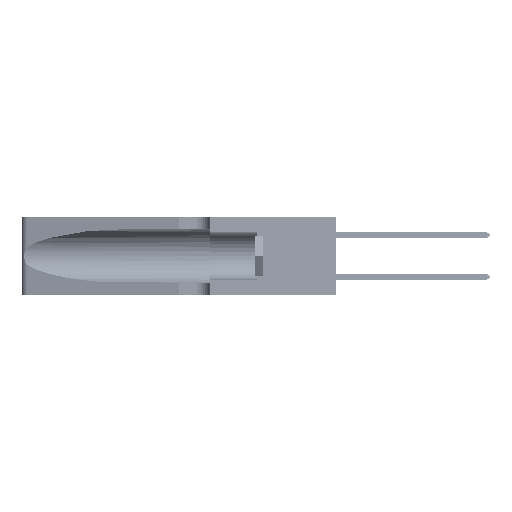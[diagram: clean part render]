
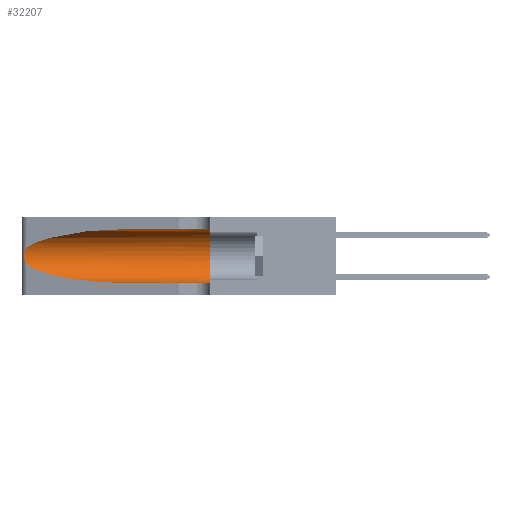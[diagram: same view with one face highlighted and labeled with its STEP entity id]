
A CAD part, left-side view. The second image highlights one B-rep face of the part: STEP entity #32207.
In plain terms, the highlighted cylindrical face has radius 3.308 mm (diameter 6.617 mm), a partial arc.
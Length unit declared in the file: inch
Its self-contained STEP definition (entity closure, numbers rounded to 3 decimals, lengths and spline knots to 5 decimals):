
#1120 = CARTESIAN_POINT ( 'NONE',  ( 0.2373, 1.15595, 0.28018 ) ) ;
#2600 = VERTEX_POINT ( 'NONE', #28276 ) ;
#2795 = EDGE_CURVE ( 'NONE', #25379, #2600, #51472, .T. ) ;
#2971 = ORIENTED_EDGE ( 'NONE', *, *, #19829, .F. ) ;
#3162 = CARTESIAN_POINT ( 'NONE',  ( 0.1305, 0.72297, 0.31525 ) ) ;
#4078 = ORIENTED_EDGE ( 'NONE', *, *, #41213, .T. ) ;
#4737 = DIRECTION ( 'NONE',  ( 0., 0., -1. ) ) ;
#5850 = CARTESIAN_POINT ( 'NONE',  ( 0.1305, 1.61858, 0.05475 ) ) ;
#6497 = CARTESIAN_POINT ( 'NONE',  ( 0.25639, 1.23184, 0.21858 ) ) ;
#6669 = CARTESIAN_POINT ( 'NONE',  ( 0.26075, 1.23896, 0.19203 ) ) ;
#8155 = CARTESIAN_POINT ( 'NONE',  ( 0.25487, 1.22718, 0.22369 ) ) ;
#8171 = CARTESIAN_POINT ( 'NONE',  ( 0.25487, 1.22718, 0.14631 ) ) ;
#10570 = CARTESIAN_POINT ( 'NONE',  ( 0.26018, 1.23835, 0.19895 ) ) ;
#12343 =( BOUNDED_CURVE ( )  B_SPLINE_CURVE ( 3, ( #16083, #21004, #1120, #45771 ),
 .UNSPECIFIED., .F., .T. ) 
 B_SPLINE_CURVE_WITH_KNOTS ( ( 4, 4 ),
 ( 1.5708, 2.84003 ),
 .UNSPECIFIED. ) 
 CURVE ( )  GEOMETRIC_REPRESENTATION_ITEM ( )  RATIONAL_B_SPLINE_CURVE ( ( 1., 0.87, 0.87, 1. ) ) 
 REPRESENTATION_ITEM ( '' )  );
#13330 = EDGE_LOOP ( 'NONE', ( #48797, #4078, #43429, #39478, #13455, #2971 ) ) ;
#13455 = ORIENTED_EDGE ( 'NONE', *, *, #2795, .F. ) ;
#14400 = CARTESIAN_POINT ( 'NONE',  ( 0.25487, 1.22718, 0.14631 ) ) ;
#14750 = CARTESIAN_POINT ( 'NONE',  ( 0.25555, 1.22994, 0.2215 ) ) ;
#14924 = CARTESIAN_POINT ( 'NONE',  ( 0.25487, 1.22718, 0.22369 ) ) ;
#16083 = CARTESIAN_POINT ( 'NONE',  ( 0.1305, 0.72297, 0.31525 ) ) ;
#17187 = VERTEX_POINT ( 'NONE', #3162 ) ;
#18982 = EDGE_CURVE ( 'NONE', #36548, #25638, #21703, .T. ) ;
#19829 = EDGE_CURVE ( 'NONE', #17187, #25379, #41629, .T. ) ;
#20240 = VECTOR ( 'NONE', #37278, 39.37008 ) ;
#20746 = DIRECTION ( 'NONE',  ( 0., 0., 1. ) ) ;
#21004 = CARTESIAN_POINT ( 'NONE',  ( 0.18966, 0.96281, 0.31525 ) ) ;
#21703 =( BOUNDED_CURVE ( )  B_SPLINE_CURVE ( 3, ( #8171, #31535, #35926, #47714 ),
 .UNSPECIFIED., .F., .F. ) 
 B_SPLINE_CURVE_WITH_KNOTS ( ( 4, 4 ),
 ( 3.44316, 4.71239 ),
 .UNSPECIFIED. ) 
 CURVE ( )  GEOMETRIC_REPRESENTATION_ITEM ( )  RATIONAL_B_SPLINE_CURVE ( ( 1., 0.87, 0.87, 1. ) ) 
 REPRESENTATION_ITEM ( '' )  );
#23038 = CARTESIAN_POINT ( 'NONE',  ( 0.25854, 1.2359, 0.20912 ) ) ;
#23856 = EDGE_CURVE ( 'NONE', #25638, #2600, #28104, .T. ) ;
#25379 = VERTEX_POINT ( 'NONE', #44426 ) ;
#25638 = VERTEX_POINT ( 'NONE', #35257 ) ;
#26495 = B_SPLINE_CURVE_WITH_KNOTS ( 'NONE', 3,
 ( #14924, #14750, #6497, #43236, #23038, #10570, #6669, #50803, #26713, #31098, #51130, #30733, #42888, #14400 ),
 .UNSPECIFIED., .F., .F.,
 ( 4, 2, 2, 2, 2, 2, 4 ),
 ( 0., 0.00027, 0.00053, 0.00107, 0.0016, 0.00187, 0.00214 ),
 .UNSPECIFIED. ) ;
#26713 = CARTESIAN_POINT ( 'NONE',  ( 0.26017, 1.23833, 0.17102 ) ) ;
#28104 = LINE ( 'NONE', #5850, #36886 ) ;
#28276 = CARTESIAN_POINT ( 'NONE',  ( 0.1305, 0.35, 0.05475 ) ) ;
#30733 = CARTESIAN_POINT ( 'NONE',  ( 0.25639, 1.23186, 0.15144 ) ) ;
#30755 = AXIS2_PLACEMENT_3D ( 'NONE', #44634, #40951, #20746 ) ;
#31098 = CARTESIAN_POINT ( 'NONE',  ( 0.25856, 1.23593, 0.16098 ) ) ;
#31535 = CARTESIAN_POINT ( 'NONE',  ( 0.2373, 1.15595, 0.08982 ) ) ;
#32207 = ADVANCED_FACE ( 'NONE', ( #48978 ), #37622, .F. ) ;
#34304 = VERTEX_POINT ( 'NONE', #8155 ) ;
#35257 = CARTESIAN_POINT ( 'NONE',  ( 0.1305, 0.72297, 0.05475 ) ) ;
#35926 = CARTESIAN_POINT ( 'NONE',  ( 0.18966, 0.96281, 0.05475 ) ) ;
#36548 = VERTEX_POINT ( 'NONE', #46779 ) ;
#36886 = VECTOR ( 'NONE', #38220, 39.37008 ) ;
#37090 = DIRECTION ( 'NONE',  ( 0., -1., 0. ) ) ;
#37278 = DIRECTION ( 'NONE',  ( 0., -1., 0. ) ) ;
#37622 = CYLINDRICAL_SURFACE ( 'NONE', #39443, 0.13025 ) ;
#38220 = DIRECTION ( 'NONE',  ( 0., -1., 0. ) ) ;
#38818 = EDGE_CURVE ( 'NONE', #17187, #34304, #12343, .T. ) ;
#39443 = AXIS2_PLACEMENT_3D ( 'NONE', #41141, #37090, #4737 ) ;
#39478 = ORIENTED_EDGE ( 'NONE', *, *, #23856, .T. ) ;
#40951 = DIRECTION ( 'NONE',  ( 0., 1., 0. ) ) ;
#41141 = CARTESIAN_POINT ( 'NONE',  ( 0.1305, 1.61858, 0.185 ) ) ;
#41213 = EDGE_CURVE ( 'NONE', #34304, #36548, #26495, .T. ) ;
#41629 = LINE ( 'NONE', #45194, #20240 ) ;
#42888 = CARTESIAN_POINT ( 'NONE',  ( 0.25555, 1.22993, 0.14849 ) ) ;
#43236 = CARTESIAN_POINT ( 'NONE',  ( 0.25787, 1.23484, 0.2124 ) ) ;
#43429 = ORIENTED_EDGE ( 'NONE', *, *, #18982, .T. ) ;
#44426 = CARTESIAN_POINT ( 'NONE',  ( 0.1305, 0.35, 0.31525 ) ) ;
#44634 = CARTESIAN_POINT ( 'NONE',  ( 0.1305, 0.35, 0.185 ) ) ;
#45194 = CARTESIAN_POINT ( 'NONE',  ( 0.1305, 1.61858, 0.31525 ) ) ;
#45771 = CARTESIAN_POINT ( 'NONE',  ( 0.25487, 1.22718, 0.22369 ) ) ;
#46779 = CARTESIAN_POINT ( 'NONE',  ( 0.25487, 1.22718, 0.14631 ) ) ;
#47714 = CARTESIAN_POINT ( 'NONE',  ( 0.1305, 0.72297, 0.05475 ) ) ;
#48797 = ORIENTED_EDGE ( 'NONE', *, *, #38818, .T. ) ;
#48978 = FACE_OUTER_BOUND ( 'NONE', #13330, .T. ) ;
#50803 = CARTESIAN_POINT ( 'NONE',  ( 0.26075, 1.23896, 0.178 ) ) ;
#51130 = CARTESIAN_POINT ( 'NONE',  ( 0.25789, 1.23486, 0.15765 ) ) ;
#51472 = CIRCLE ( 'NONE', #30755, 0.13025 ) ;
